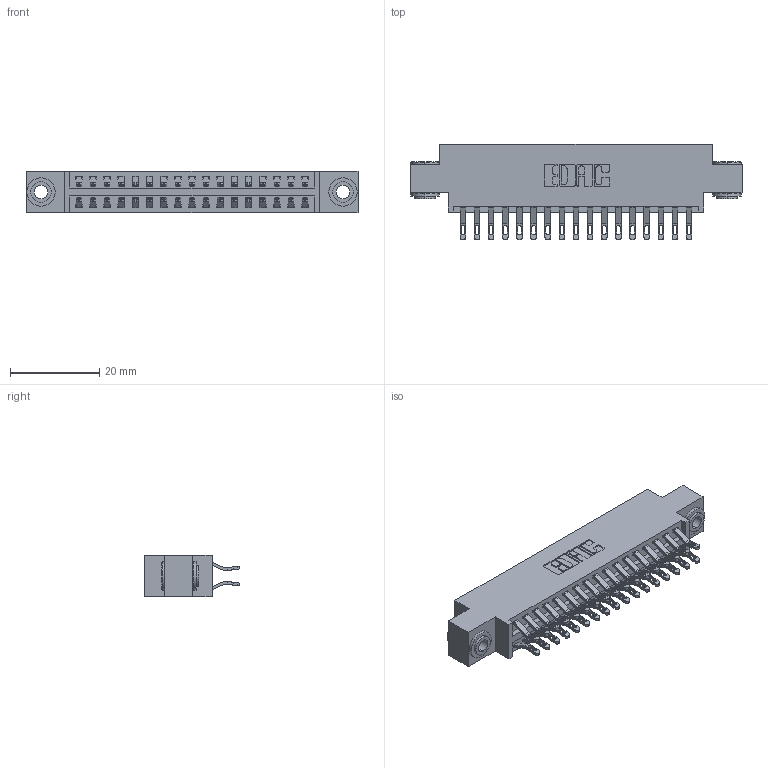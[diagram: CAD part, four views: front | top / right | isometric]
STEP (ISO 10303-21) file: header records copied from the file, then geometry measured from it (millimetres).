
FILE_DESCRIPTION (( 'STEP AP203' ), '1' );
FILE_NAME ('346-034-555-803.STEP', '2022-05-19T20:04:10', ( '' ), ( '' ), 'SwSTEP 2.0', 'SolidWorks 2020', '' );
FILE_SCHEMA (( 'CONFIG_CONTROL_DESIGN' ));
Length unit declared in the file: inch
Products named in the file (4): 346-034-555-803; 345-250-002_345-250-002-102; 345-292-001_555 Tail; 346 Part_0.170 Offset - 0.156 Dia-TH
Assembly tree (37 placements, depth 2):
  346-034-555-803
    346 Part_0.170 Offset - 0.156 Dia-TH
    345-292-001_555 Tail  x34
    345-250-002_345-250-002-102  x2
Bounding box: 74.55 x 21.46 x 9.4 mm (x, y, z)
Volume: 7020.6 mm3; surface area: 10037.2 mm2
Topology: 37 solids, 37 shells, 2150 faces, 6675 edges, 4446 vertices
Faces by surface type: plane 1226, cylinder 916, cone 8
Entity records: 15984 total; most frequent: CARTESIAN_POINT 2687, ORIENTED_EDGE 2582, DIRECTION 2417, EDGE_CURVE 1291, VECTOR 1047, LINE 1047, VERTEX_POINT 858, AXIS2_PLACEMENT_3D 685
